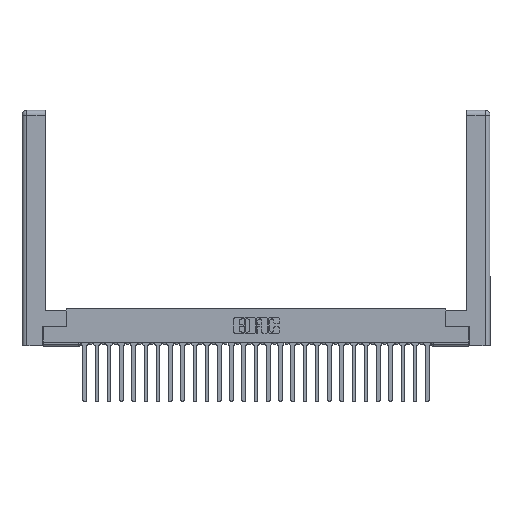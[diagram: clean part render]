
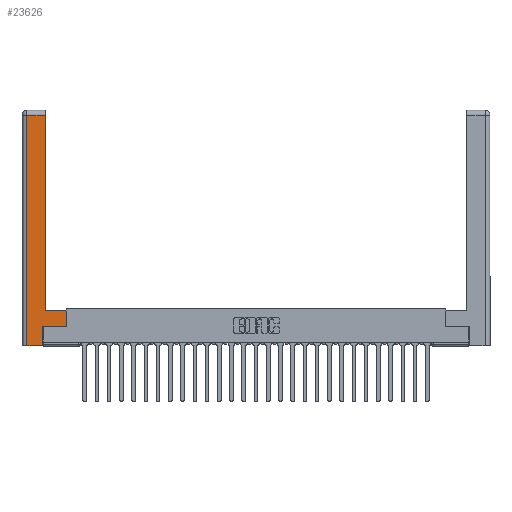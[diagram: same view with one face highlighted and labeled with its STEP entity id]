
A CAD part, top view. The second image highlights one B-rep face of the part: STEP entity #23626.
In plain terms, the highlighted planar face has unit normal (0, 0, 1).
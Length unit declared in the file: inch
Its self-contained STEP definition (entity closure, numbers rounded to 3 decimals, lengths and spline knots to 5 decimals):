
#267 = VERTEX_POINT ( 'NONE', #8542 ) ;
#282 = ORIENTED_EDGE ( 'NONE', *, *, #28667, .T. ) ;
#841 = VECTOR ( 'NONE', #9481, 39.37008 ) ;
#1321 = VECTOR ( 'NONE', #3107, 39.37008 ) ;
#2322 = PLANE ( 'NONE',  #9293 ) ;
#2603 = ORIENTED_EDGE ( 'NONE', *, *, #25675, .T. ) ;
#3107 = DIRECTION ( 'NONE',  ( -1., 0., 0. ) ) ;
#3723 = ORIENTED_EDGE ( 'NONE', *, *, #24273, .T. ) ;
#4492 = CARTESIAN_POINT ( 'NONE',  ( 0.265, 0., 0. ) ) ;
#4624 = CARTESIAN_POINT ( 'NONE',  ( 0., 0., 0. ) ) ;
#4740 = CARTESIAN_POINT ( 'NONE',  ( 0.565, 0.45, 0. ) ) ;
#4989 = CARTESIAN_POINT ( 'NONE',  ( 0.565, 0.245, 0. ) ) ;
#5243 = EDGE_CURVE ( 'NONE', #17730, #27901, #7862, .T. ) ;
#5340 = CARTESIAN_POINT ( 'NONE',  ( 0.265, 0.245, 0. ) ) ;
#5747 = EDGE_LOOP ( 'NONE', ( #27684, #8624, #14986, #19886, #282, #3723, #29299, #2603 ) ) ;
#5968 = CARTESIAN_POINT ( 'NONE',  ( 0.565, 0.45, 0. ) ) ;
#7225 = CARTESIAN_POINT ( 'NONE',  ( 0.295, 0.45, 0. ) ) ;
#7792 = EDGE_CURVE ( 'NONE', #27901, #267, #24438, .T. ) ;
#7804 = VECTOR ( 'NONE', #25790, 39.37008 ) ;
#7862 = LINE ( 'NONE', #10193, #25628 ) ;
#8542 = CARTESIAN_POINT ( 'NONE',  ( 0.0615, 2.94, 0. ) ) ;
#8624 = ORIENTED_EDGE ( 'NONE', *, *, #7792, .T. ) ;
#8917 = VECTOR ( 'NONE', #18593, 39.37008 ) ;
#9293 = AXIS2_PLACEMENT_3D ( 'NONE', #4624, #25625, #23220 ) ;
#9481 = DIRECTION ( 'NONE',  ( 0., 1., 0. ) ) ;
#10193 = CARTESIAN_POINT ( 'NONE',  ( 0.295, 3., 0. ) ) ;
#10320 = CARTESIAN_POINT ( 'NONE',  ( 0.565, 0.245, 0. ) ) ;
#10915 = VERTEX_POINT ( 'NONE', #17426 ) ;
#11032 = LINE ( 'NONE', #13787, #28095 ) ;
#12517 = CARTESIAN_POINT ( 'NONE',  ( 0.295, 2.94, 0. ) ) ;
#12595 = VECTOR ( 'NONE', #13848, 39.37008 ) ;
#12677 = CARTESIAN_POINT ( 'NONE',  ( 0.0615, 0., 0. ) ) ;
#13787 = CARTESIAN_POINT ( 'NONE',  ( 0.0615, 0., 0. ) ) ;
#13848 = DIRECTION ( 'NONE',  ( 0., 1., 0. ) ) ;
#14169 = VERTEX_POINT ( 'NONE', #12677 ) ;
#14986 = ORIENTED_EDGE ( 'NONE', *, *, #19756, .T. ) ;
#15127 = LINE ( 'NONE', #4492, #8917 ) ;
#15910 = VERTEX_POINT ( 'NONE', #10320 ) ;
#17426 = CARTESIAN_POINT ( 'NONE',  ( 0.265, 0., 0. ) ) ;
#17730 = VERTEX_POINT ( 'NONE', #7225 ) ;
#17982 = LINE ( 'NONE', #21263, #1321 ) ;
#18593 = DIRECTION ( 'NONE',  ( 1., 0., 0. ) ) ;
#19756 = EDGE_CURVE ( 'NONE', #267, #14169, #11032, .T. ) ;
#19886 = ORIENTED_EDGE ( 'NONE', *, *, #29847, .T. ) ;
#19931 = LINE ( 'NONE', #23544, #12595 ) ;
#20938 = DIRECTION ( 'NONE',  ( -1., 0., 0. ) ) ;
#21263 = CARTESIAN_POINT ( 'NONE',  ( 0.295, 0.45, 0. ) ) ;
#21532 = VECTOR ( 'NONE', #20938, 39.37008 ) ;
#21597 = FACE_OUTER_BOUND ( 'NONE', #5747, .T. ) ;
#21911 = EDGE_CURVE ( 'NONE', #15910, #23983, #27969, .T. ) ;
#23220 = DIRECTION ( 'NONE',  ( -1., 0., 0. ) ) ;
#23544 = CARTESIAN_POINT ( 'NONE',  ( 0.265, 0.245, 0. ) ) ;
#23626 = ADVANCED_FACE ( 'NONE', ( #21597 ), #2322, .F. ) ;
#23983 = VERTEX_POINT ( 'NONE', #5968 ) ;
#24273 = EDGE_CURVE ( 'NONE', #27930, #15910, #27064, .T. ) ;
#24438 = LINE ( 'NONE', #25587, #21532 ) ;
#25587 = CARTESIAN_POINT ( 'NONE',  ( 0.0615, 2.94, 0. ) ) ;
#25625 = DIRECTION ( 'NONE',  ( 0., 0., -1. ) ) ;
#25628 = VECTOR ( 'NONE', #28690, 39.37008 ) ;
#25675 = EDGE_CURVE ( 'NONE', #23983, #17730, #17982, .T. ) ;
#25790 = DIRECTION ( 'NONE',  ( 1., 0., 0. ) ) ;
#27064 = LINE ( 'NONE', #4989, #7804 ) ;
#27684 = ORIENTED_EDGE ( 'NONE', *, *, #5243, .T. ) ;
#27901 = VERTEX_POINT ( 'NONE', #12517 ) ;
#27930 = VERTEX_POINT ( 'NONE', #5340 ) ;
#27969 = LINE ( 'NONE', #4740, #841 ) ;
#28018 = DIRECTION ( 'NONE',  ( 0., -1., 0. ) ) ;
#28095 = VECTOR ( 'NONE', #28018, 39.37008 ) ;
#28667 = EDGE_CURVE ( 'NONE', #10915, #27930, #19931, .T. ) ;
#28690 = DIRECTION ( 'NONE',  ( 0., 1., 0. ) ) ;
#29299 = ORIENTED_EDGE ( 'NONE', *, *, #21911, .T. ) ;
#29847 = EDGE_CURVE ( 'NONE', #14169, #10915, #15127, .T. ) ;
